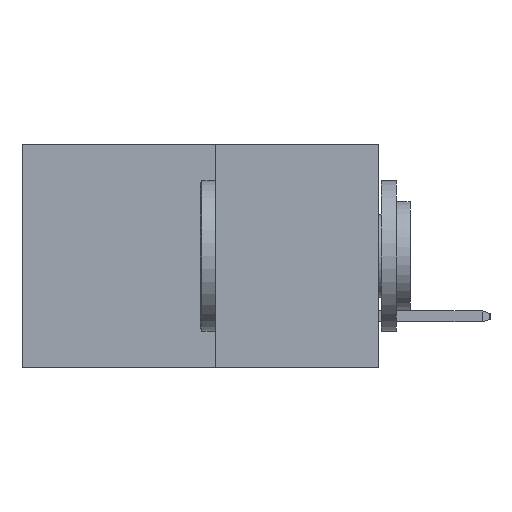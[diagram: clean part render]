
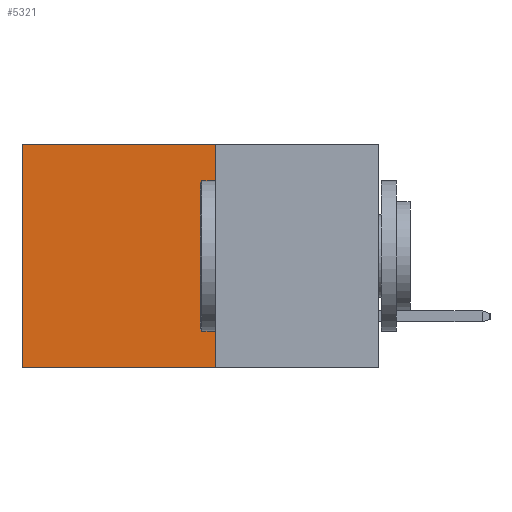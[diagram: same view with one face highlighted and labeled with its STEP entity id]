
A CAD part, left-side view. The second image highlights one B-rep face of the part: STEP entity #5321.
In plain terms, the highlighted planar face has unit normal (-1, 0, 0).
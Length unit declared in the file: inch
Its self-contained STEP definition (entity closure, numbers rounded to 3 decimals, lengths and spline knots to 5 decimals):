
#204 = CARTESIAN_POINT ( 'NONE',  ( 0.277, 0.27, 0. ) ) ;
#993 = CARTESIAN_POINT ( 'NONE',  ( 0.277, 0.59, -0.37 ) ) ;
#1296 = ORIENTED_EDGE ( 'NONE', *, *, #9965, .T. ) ;
#1529 = LINE ( 'NONE', #204, #4064 ) ;
#2246 = EDGE_CURVE ( 'NONE', #5474, #6829, #1529, .T. ) ;
#2509 = EDGE_CURVE ( 'NONE', #9672, #9331, #11702, .T. ) ;
#2736 = VECTOR ( 'NONE', #10385, 39.37008 ) ;
#2969 = DIRECTION ( 'NONE',  ( 0., 1., 0. ) ) ;
#3052 = CARTESIAN_POINT ( 'NONE',  ( 0.277, 0.27, -0.37 ) ) ;
#3683 = DIRECTION ( 'NONE',  ( 0., 0., -1. ) ) ;
#4064 = VECTOR ( 'NONE', #12363, 39.37008 ) ;
#4950 = EDGE_CURVE ( 'NONE', #5474, #9672, #11510, .T. ) ;
#5321 = ADVANCED_FACE ( 'NONE', ( #7094 ), #7831, .F. ) ;
#5474 = VERTEX_POINT ( 'NONE', #12014 ) ;
#5609 = CARTESIAN_POINT ( 'NONE',  ( 0.277, 0.59, 0. ) ) ;
#5920 = AXIS2_PLACEMENT_3D ( 'NONE', #6796, #9872, #3683 ) ;
#6075 = ORIENTED_EDGE ( 'NONE', *, *, #2246, .T. ) ;
#6138 = VECTOR ( 'NONE', #6580, 39.37008 ) ;
#6580 = DIRECTION ( 'NONE',  ( 0., 0., -1. ) ) ;
#6666 = VECTOR ( 'NONE', #2969, 39.37008 ) ;
#6796 = CARTESIAN_POINT ( 'NONE',  ( 0.277, 0.27, -0.37 ) ) ;
#6829 = VERTEX_POINT ( 'NONE', #5609 ) ;
#7094 = FACE_OUTER_BOUND ( 'NONE', #12662, .T. ) ;
#7535 = CARTESIAN_POINT ( 'NONE',  ( 0.277, 0.27, -0.37 ) ) ;
#7831 = PLANE ( 'NONE',  #5920 ) ;
#8493 = CARTESIAN_POINT ( 'NONE',  ( 0.277, 0.59, -0.37 ) ) ;
#9331 = VERTEX_POINT ( 'NONE', #8493 ) ;
#9672 = VERTEX_POINT ( 'NONE', #9740 ) ;
#9740 = CARTESIAN_POINT ( 'NONE',  ( 0.277, 0.27, -0.37 ) ) ;
#9872 = DIRECTION ( 'NONE',  ( 1., 0., 0. ) ) ;
#9965 = EDGE_CURVE ( 'NONE', #6829, #9331, #10988, .T. ) ;
#10385 = DIRECTION ( 'NONE',  ( 0., 0., -1. ) ) ;
#10704 = ORIENTED_EDGE ( 'NONE', *, *, #4950, .F. ) ;
#10988 = LINE ( 'NONE', #993, #2736 ) ;
#11189 = ORIENTED_EDGE ( 'NONE', *, *, #2509, .F. ) ;
#11510 = LINE ( 'NONE', #7535, #6138 ) ;
#11702 = LINE ( 'NONE', #3052, #6666 ) ;
#12014 = CARTESIAN_POINT ( 'NONE',  ( 0.277, 0.27, 0. ) ) ;
#12363 = DIRECTION ( 'NONE',  ( 0., 1., 0. ) ) ;
#12662 = EDGE_LOOP ( 'NONE', ( #1296, #11189, #10704, #6075 ) ) ;
